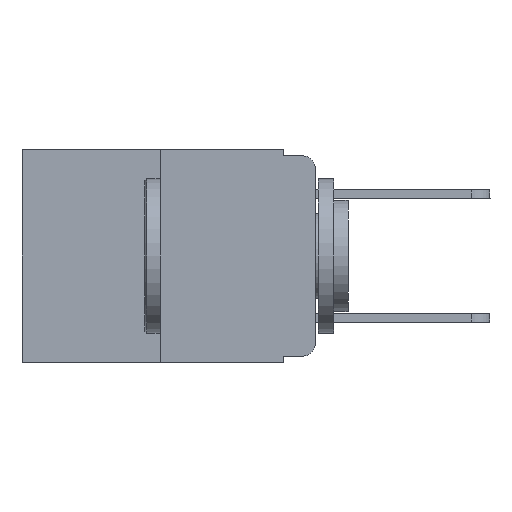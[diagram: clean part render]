
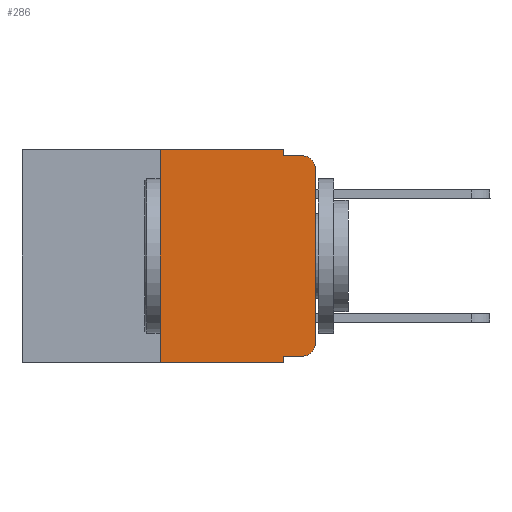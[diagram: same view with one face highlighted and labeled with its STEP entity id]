
A CAD part, left-side view. The second image highlights one B-rep face of the part: STEP entity #286.
In plain terms, the highlighted planar face has unit normal (-1, 0, 0).
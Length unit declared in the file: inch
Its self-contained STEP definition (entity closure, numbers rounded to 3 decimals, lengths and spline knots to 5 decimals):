
#286 = ADVANCED_FACE ( 'NONE', ( #8986 ), #1245, .F. ) ;
#488 = ORIENTED_EDGE ( 'NONE', *, *, #5319, .T. ) ;
#540 = VERTEX_POINT ( 'NONE', #7530 ) ;
#655 = VERTEX_POINT ( 'NONE', #8064 ) ;
#773 = EDGE_CURVE ( 'NONE', #6280, #8155, #9883, .T. ) ;
#794 = LINE ( 'NONE', #6622, #4448 ) ;
#796 = DIRECTION ( 'NONE',  ( 0., -1., 0. ) ) ;
#844 = ORIENTED_EDGE ( 'NONE', *, *, #3519, .F. ) ;
#871 = VECTOR ( 'NONE', #3885, 39.37008 ) ;
#1093 = CARTESIAN_POINT ( 'NONE',  ( 0., 0.473, 0. ) ) ;
#1124 = EDGE_CURVE ( 'NONE', #540, #3279, #4804, .T. ) ;
#1245 = PLANE ( 'NONE',  #6867 ) ;
#1593 = VECTOR ( 'NONE', #3309, 39.37008 ) ;
#2037 = CARTESIAN_POINT ( 'NONE',  ( 0., 0.02, -0.01 ) ) ;
#2107 = VECTOR ( 'NONE', #6870, 39.37008 ) ;
#2210 = CARTESIAN_POINT ( 'NONE',  ( 0., 0.02, -0.313 ) ) ;
#2318 = CIRCLE ( 'NONE', #3926, 0.02 ) ;
#2461 = DIRECTION ( 'NONE',  ( 0., -1., 0. ) ) ;
#2478 = CARTESIAN_POINT ( 'NONE',  ( 0., 0., 0. ) ) ;
#2509 = DIRECTION ( 'NONE',  ( 0., 0., 1. ) ) ;
#2541 = DIRECTION ( 'NONE',  ( 0., -1., 0. ) ) ;
#2819 = ORIENTED_EDGE ( 'NONE', *, *, #7234, .T. ) ;
#2860 = VECTOR ( 'NONE', #2461, 39.37008 ) ;
#3005 = ORIENTED_EDGE ( 'NONE', *, *, #5844, .F. ) ;
#3194 = CARTESIAN_POINT ( 'NONE',  ( 0., 0.473, 0. ) ) ;
#3225 = VECTOR ( 'NONE', #2509, 39.37008 ) ;
#3279 = VERTEX_POINT ( 'NONE', #9605 ) ;
#3309 = DIRECTION ( 'NONE',  ( 0., 0., 1. ) ) ;
#3519 = EDGE_CURVE ( 'NONE', #5433, #10803, #8786, .T. ) ;
#3538 = ORIENTED_EDGE ( 'NONE', *, *, #1124, .F. ) ;
#3803 = ORIENTED_EDGE ( 'NONE', *, *, #8958, .T. ) ;
#3861 = CARTESIAN_POINT ( 'NONE',  ( 0., 0., -0.313 ) ) ;
#3885 = DIRECTION ( 'NONE',  ( 0., 0., -1. ) ) ;
#3906 = LINE ( 'NONE', #3194, #8104 ) ;
#3926 = AXIS2_PLACEMENT_3D ( 'NONE', #8630, #5228, #7807 ) ;
#4305 = CIRCLE ( 'NONE', #6612, 0.02 ) ;
#4376 = CARTESIAN_POINT ( 'NONE',  ( 0., 0.25, -0.343 ) ) ;
#4448 = VECTOR ( 'NONE', #796, 39.37008 ) ;
#4714 = LINE ( 'NONE', #6112, #2107 ) ;
#4803 = EDGE_LOOP ( 'NONE', ( #9994, #3803, #9353, #3538, #3005, #844, #5505, #6812, #488, #2819 ) ) ;
#4804 = LINE ( 'NONE', #8069, #871 ) ;
#4808 = CARTESIAN_POINT ( 'NONE',  ( 0., 0.25, 0. ) ) ;
#4972 = CARTESIAN_POINT ( 'NONE',  ( 0., 0.25, 0. ) ) ;
#5228 = DIRECTION ( 'NONE',  ( -1., 0., 0. ) ) ;
#5291 = DIRECTION ( 'NONE',  ( 1., 0., 0. ) ) ;
#5319 = EDGE_CURVE ( 'NONE', #655, #7413, #794, .T. ) ;
#5433 = VERTEX_POINT ( 'NONE', #4376 ) ;
#5470 = CARTESIAN_POINT ( 'NONE',  ( 0., 0.051, -0.343 ) ) ;
#5505 = ORIENTED_EDGE ( 'NONE', *, *, #10519, .T. ) ;
#5566 = DIRECTION ( 'NONE',  ( -1., 0., 0. ) ) ;
#5844 = EDGE_CURVE ( 'NONE', #10803, #540, #3906, .T. ) ;
#5967 = LINE ( 'NONE', #9977, #9590 ) ;
#6112 = CARTESIAN_POINT ( 'NONE',  ( 0., 0.051, 0. ) ) ;
#6165 = LINE ( 'NONE', #10809, #2860 ) ;
#6280 = VERTEX_POINT ( 'NONE', #3861 ) ;
#6581 = CARTESIAN_POINT ( 'NONE',  ( 0., 0., -0.03 ) ) ;
#6612 = AXIS2_PLACEMENT_3D ( 'NONE', #2210, #5566, #8873 ) ;
#6622 = CARTESIAN_POINT ( 'NONE',  ( 0., 0.051, -0.333 ) ) ;
#6646 = VERTEX_POINT ( 'NONE', #5470 ) ;
#6812 = ORIENTED_EDGE ( 'NONE', *, *, #7018, .F. ) ;
#6867 = AXIS2_PLACEMENT_3D ( 'NONE', #1093, #5291, #7759 ) ;
#6870 = DIRECTION ( 'NONE',  ( 0., 0., -1. ) ) ;
#7018 = EDGE_CURVE ( 'NONE', #655, #6646, #4714, .T. ) ;
#7234 = EDGE_CURVE ( 'NONE', #7413, #6280, #4305, .T. ) ;
#7413 = VERTEX_POINT ( 'NONE', #8018 ) ;
#7530 = CARTESIAN_POINT ( 'NONE',  ( 0., 0.051, 0. ) ) ;
#7551 = EDGE_CURVE ( 'NONE', #3279, #10578, #6165, .T. ) ;
#7759 = DIRECTION ( 'NONE',  ( 0., 0., -1. ) ) ;
#7807 = DIRECTION ( 'NONE',  ( 0., 0., -1. ) ) ;
#8018 = CARTESIAN_POINT ( 'NONE',  ( 0., 0.02, -0.333 ) ) ;
#8064 = CARTESIAN_POINT ( 'NONE',  ( 0., 0.051, -0.333 ) ) ;
#8069 = CARTESIAN_POINT ( 'NONE',  ( 0., 0.051, 0. ) ) ;
#8104 = VECTOR ( 'NONE', #8205, 39.37008 ) ;
#8155 = VERTEX_POINT ( 'NONE', #6581 ) ;
#8205 = DIRECTION ( 'NONE',  ( 0., -1., 0. ) ) ;
#8630 = CARTESIAN_POINT ( 'NONE',  ( 0., 0.02, -0.03 ) ) ;
#8786 = LINE ( 'NONE', #4972, #1593 ) ;
#8873 = DIRECTION ( 'NONE',  ( 0., 0., -1. ) ) ;
#8958 = EDGE_CURVE ( 'NONE', #8155, #10578, #2318, .T. ) ;
#8986 = FACE_OUTER_BOUND ( 'NONE', #4803, .T. ) ;
#9353 = ORIENTED_EDGE ( 'NONE', *, *, #7551, .F. ) ;
#9590 = VECTOR ( 'NONE', #2541, 39.37008 ) ;
#9605 = CARTESIAN_POINT ( 'NONE',  ( 0., 0.051, -0.01 ) ) ;
#9883 = LINE ( 'NONE', #2478, #3225 ) ;
#9977 = CARTESIAN_POINT ( 'NONE',  ( 0., 0.473, -0.343 ) ) ;
#9994 = ORIENTED_EDGE ( 'NONE', *, *, #773, .T. ) ;
#10519 = EDGE_CURVE ( 'NONE', #5433, #6646, #5967, .T. ) ;
#10578 = VERTEX_POINT ( 'NONE', #2037 ) ;
#10803 = VERTEX_POINT ( 'NONE', #4808 ) ;
#10809 = CARTESIAN_POINT ( 'NONE',  ( 0., 0.051, -0.01 ) ) ;
